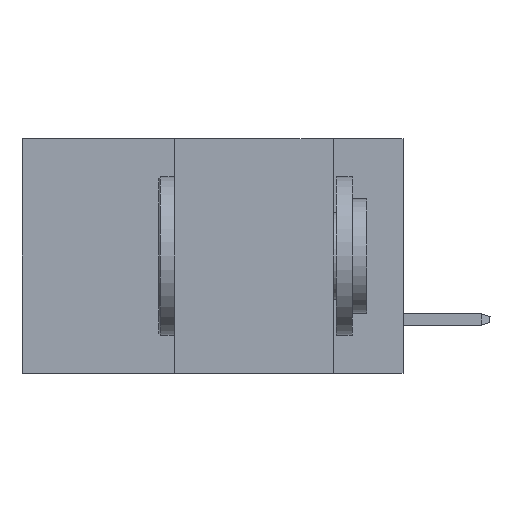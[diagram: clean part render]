
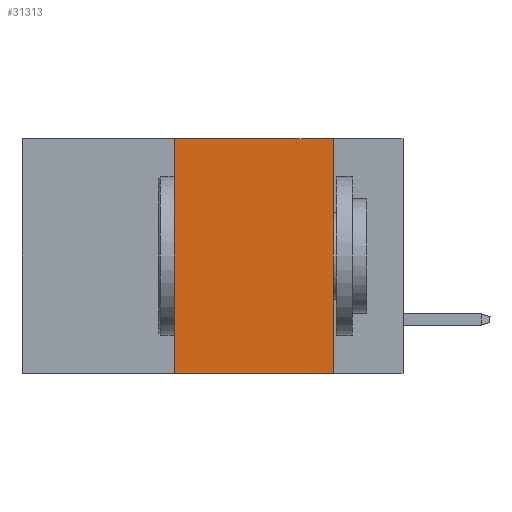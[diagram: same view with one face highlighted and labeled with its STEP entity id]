
A CAD part, left-side view. The second image highlights one B-rep face of the part: STEP entity #31313.
In plain terms, the highlighted planar face has unit normal (-1, 0, 0).
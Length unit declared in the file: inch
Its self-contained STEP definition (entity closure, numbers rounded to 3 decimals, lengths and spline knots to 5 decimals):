
#510 = VECTOR ( 'NONE', #3689, 39.37008 ) ;
#3500 = VECTOR ( 'NONE', #16959, 39.37008 ) ;
#3689 = DIRECTION ( 'NONE',  ( 0., -1., 0. ) ) ;
#3744 = VERTEX_POINT ( 'NONE', #5945 ) ;
#5274 = CARTESIAN_POINT ( 'NONE',  ( 0., 0.36, 0. ) ) ;
#5945 = CARTESIAN_POINT ( 'NONE',  ( 0., 0.11, 0. ) ) ;
#6165 = LINE ( 'NONE', #16790, #3500 ) ;
#6644 = EDGE_CURVE ( 'NONE', #3744, #31787, #34458, .T. ) ;
#6715 = DIRECTION ( 'NONE',  ( 0., 0., -1. ) ) ;
#8852 = CARTESIAN_POINT ( 'NONE',  ( 0., 0.36, -0.37 ) ) ;
#10162 = ORIENTED_EDGE ( 'NONE', *, *, #6644, .F. ) ;
#14992 = CARTESIAN_POINT ( 'NONE',  ( 0., 0.6, 0. ) ) ;
#16790 = CARTESIAN_POINT ( 'NONE',  ( 0., 0.6, 0. ) ) ;
#16959 = DIRECTION ( 'NONE',  ( 0., -1., 0. ) ) ;
#17928 = DIRECTION ( 'NONE',  ( 0., 0., -1. ) ) ;
#18649 = AXIS2_PLACEMENT_3D ( 'NONE', #14992, #20557, #6715 ) ;
#18717 = EDGE_CURVE ( 'NONE', #28053, #27078, #24505, .T. ) ;
#20557 = DIRECTION ( 'NONE',  ( 1., 0., 0. ) ) ;
#21583 = ORIENTED_EDGE ( 'NONE', *, *, #18717, .F. ) ;
#22294 = VECTOR ( 'NONE', #17928, 39.37008 ) ;
#22552 = FACE_OUTER_BOUND ( 'NONE', #30777, .T. ) ;
#23014 = EDGE_CURVE ( 'NONE', #28053, #31787, #27974, .T. ) ;
#23774 = ORIENTED_EDGE ( 'NONE', *, *, #26868, .F. ) ;
#24505 = LINE ( 'NONE', #5274, #34184 ) ;
#26868 = EDGE_CURVE ( 'NONE', #27078, #3744, #6165, .T. ) ;
#27078 = VERTEX_POINT ( 'NONE', #32578 ) ;
#27974 = LINE ( 'NONE', #30873, #510 ) ;
#28053 = VERTEX_POINT ( 'NONE', #8852 ) ;
#28132 = PLANE ( 'NONE',  #18649 ) ;
#28399 = DIRECTION ( 'NONE',  ( 0., 0., 1. ) ) ;
#30664 = ORIENTED_EDGE ( 'NONE', *, *, #23014, .T. ) ;
#30777 = EDGE_LOOP ( 'NONE', ( #10162, #23774, #21583, #30664 ) ) ;
#30873 = CARTESIAN_POINT ( 'NONE',  ( 0., 0.6, -0.37 ) ) ;
#31313 = ADVANCED_FACE ( 'NONE', ( #22552 ), #28132, .F. ) ;
#31412 = CARTESIAN_POINT ( 'NONE',  ( 0., 0.11, 0. ) ) ;
#31787 = VERTEX_POINT ( 'NONE', #34174 ) ;
#32578 = CARTESIAN_POINT ( 'NONE',  ( 0., 0.36, 0. ) ) ;
#34174 = CARTESIAN_POINT ( 'NONE',  ( 0., 0.11, -0.37 ) ) ;
#34184 = VECTOR ( 'NONE', #28399, 39.37008 ) ;
#34458 = LINE ( 'NONE', #31412, #22294 ) ;
